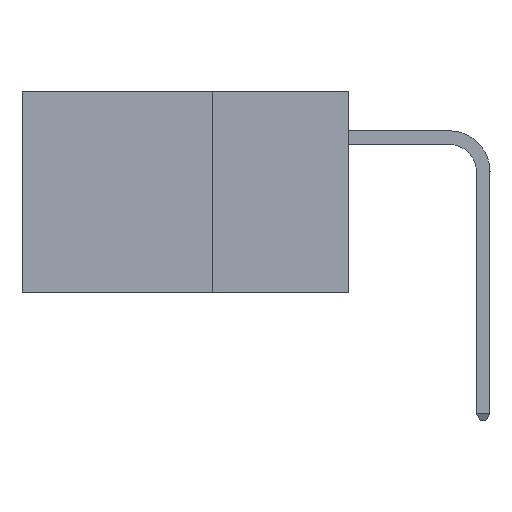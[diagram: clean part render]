
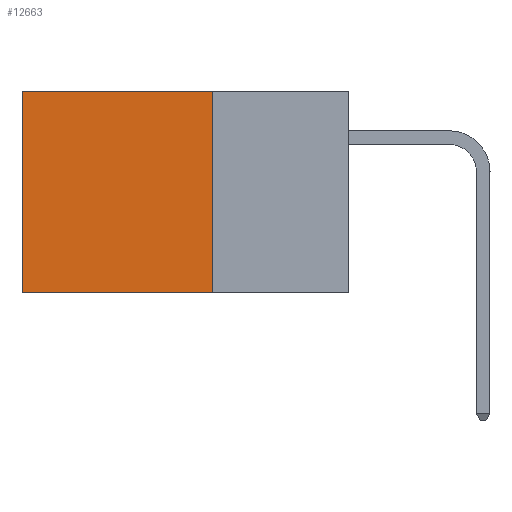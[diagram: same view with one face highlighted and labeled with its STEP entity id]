
A CAD part, left-side view. The second image highlights one B-rep face of the part: STEP entity #12663.
In plain terms, the highlighted planar face has unit normal (-1, 0, 0).
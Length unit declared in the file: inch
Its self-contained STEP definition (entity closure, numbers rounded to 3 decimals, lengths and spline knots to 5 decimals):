
#139 = LINE ( 'NONE', #1161, #11252 ) ;
#838 = EDGE_CURVE ( 'NONE', #17076, #3073, #11095, .T. ) ;
#1161 = CARTESIAN_POINT ( 'NONE',  ( 0.2875, 0.25, 0. ) ) ;
#1372 = DIRECTION ( 'NONE',  ( 0., 0., -1. ) ) ;
#1606 = CARTESIAN_POINT ( 'NONE',  ( 0.2875, 0.6, -0.37 ) ) ;
#1916 = CARTESIAN_POINT ( 'NONE',  ( 0.2875, 0.25, -0.37 ) ) ;
#2099 = CARTESIAN_POINT ( 'NONE',  ( 0.2875, 0.25, -0.37 ) ) ;
#2388 = VERTEX_POINT ( 'NONE', #13288 ) ;
#2422 = VECTOR ( 'NONE', #5091, 39.37008 ) ;
#2815 = EDGE_LOOP ( 'NONE', ( #17374, #12484, #15567, #5494 ) ) ;
#3073 = VERTEX_POINT ( 'NONE', #1916 ) ;
#3235 = EDGE_CURVE ( 'NONE', #2388, #13224, #11857, .T. ) ;
#4102 = CARTESIAN_POINT ( 'NONE',  ( 0.2875, 0.25, 0. ) ) ;
#4621 = DIRECTION ( 'NONE',  ( 0., 0., -1. ) ) ;
#5091 = DIRECTION ( 'NONE',  ( 0., 1., 0. ) ) ;
#5494 = ORIENTED_EDGE ( 'NONE', *, *, #10307, .T. ) ;
#6674 = CARTESIAN_POINT ( 'NONE',  ( 0.2875, 0.25, 0. ) ) ;
#8127 = FACE_OUTER_BOUND ( 'NONE', #2815, .T. ) ;
#8649 = CARTESIAN_POINT ( 'NONE',  ( 0.2875, 0.25, 0. ) ) ;
#8764 = DIRECTION ( 'NONE',  ( 1., 0., 0. ) ) ;
#9535 = AXIS2_PLACEMENT_3D ( 'NONE', #8649, #8764, #4621 ) ;
#10307 = EDGE_CURVE ( 'NONE', #17076, #2388, #139, .T. ) ;
#11095 = LINE ( 'NONE', #6674, #16337 ) ;
#11252 = VECTOR ( 'NONE', #15203, 39.37008 ) ;
#11396 = PLANE ( 'NONE',  #9535 ) ;
#11637 = VECTOR ( 'NONE', #16383, 39.37008 ) ;
#11857 = LINE ( 'NONE', #13579, #11637 ) ;
#12484 = ORIENTED_EDGE ( 'NONE', *, *, #12956, .F. ) ;
#12663 = ADVANCED_FACE ( 'NONE', ( #8127 ), #11396, .F. ) ;
#12956 = EDGE_CURVE ( 'NONE', #3073, #13224, #13570, .T. ) ;
#13224 = VERTEX_POINT ( 'NONE', #1606 ) ;
#13288 = CARTESIAN_POINT ( 'NONE',  ( 0.2875, 0.6, 0. ) ) ;
#13570 = LINE ( 'NONE', #2099, #2422 ) ;
#13579 = CARTESIAN_POINT ( 'NONE',  ( 0.2875, 0.6, 0. ) ) ;
#15203 = DIRECTION ( 'NONE',  ( 0., 1., 0. ) ) ;
#15567 = ORIENTED_EDGE ( 'NONE', *, *, #838, .F. ) ;
#16337 = VECTOR ( 'NONE', #1372, 39.37008 ) ;
#16383 = DIRECTION ( 'NONE',  ( 0., 0., -1. ) ) ;
#17076 = VERTEX_POINT ( 'NONE', #4102 ) ;
#17374 = ORIENTED_EDGE ( 'NONE', *, *, #3235, .T. ) ;
